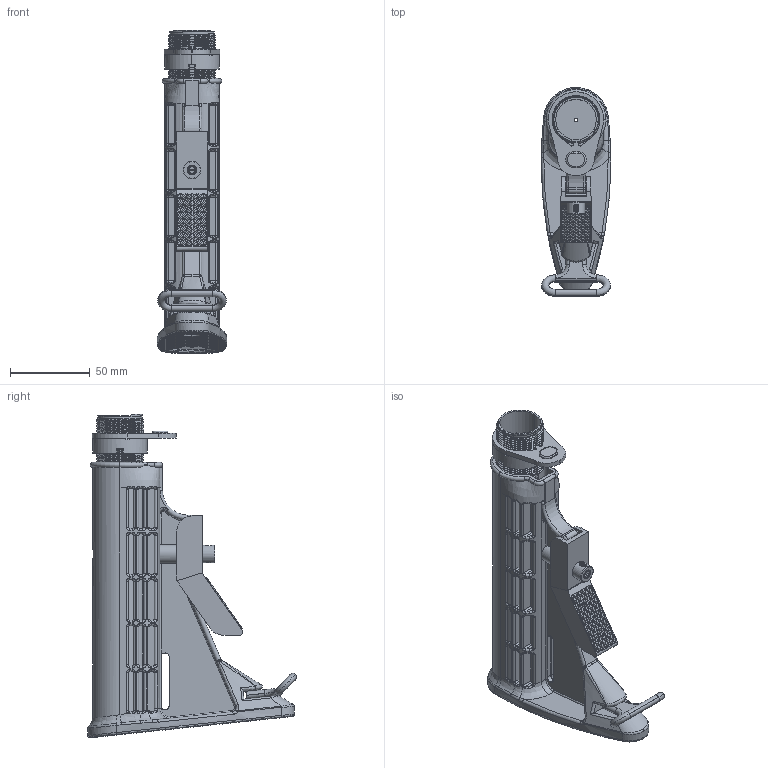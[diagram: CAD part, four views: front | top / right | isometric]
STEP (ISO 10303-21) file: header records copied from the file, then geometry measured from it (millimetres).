
FILE_DESCRIPTION (( 'STEP AP214' ), '1' );
FILE_NAME ('User Library-Telescopic Stock_1.STEP', '2013-05-22T15:48:38', ( 'Asher' ), ( '' ), 'SwSTEP 2.0', 'SolidWorks 2013', '' );
FILE_SCHEMA (( 'AUTOMOTIVE_DESIGN' ));
Length unit declared in the file: inch
Products named in the file (12): User Library-Telescopic Stock_Telescopic Stock Tube1_1; User Library-Telescopic Stock_Telescopic Stock Swivel Screw1_1; User Library-Telescopic Stock_Stock Bolt1_1; User Library-Telescopic Stock_Telescopic Stock Spring_Installed1_1; User Library-Telescopic Stock_1; User Library-Telescopic Stock_Stock Bolt Nut1_1; User Library-Telescopic Stock_Telescopic Stock Swivel1_1; User Library-Telescopic Stock_5310-917-1154_1; User Library-Telescopic Stock_Telescopic Stock_Default_As Machined_1_1; User Library-Telescopic Stock_Telescopic stock Roll Pin1_1; User Library-Telescopic Stock_Telescopic Stock Lever1_1; User Library-Telescopic Stock_1005-914-2943_1
Assembly tree (11 placements, depth 2):
  User Library-Telescopic Stock_1
    User Library-Telescopic Stock_Telescopic Stock Spring_Installed1_1
    User Library-Telescopic Stock_Stock Bolt1_1
    User Library-Telescopic Stock_Telescopic Stock Swivel Screw1_1
    User Library-Telescopic Stock_Telescopic Stock Tube1_1
    User Library-Telescopic Stock_1005-914-2943_1
    User Library-Telescopic Stock_Telescopic Stock Lever1_1
    User Library-Telescopic Stock_Telescopic stock Roll Pin1_1
    User Library-Telescopic Stock_Telescopic Stock_Default_As Machined_1_1
    User Library-Telescopic Stock_5310-917-1154_1
    User Library-Telescopic Stock_Telescopic Stock Swivel1_1
    User Library-Telescopic Stock_Stock Bolt Nut1_1
Bounding box: 43.56 x 130.88 x 202.7 mm (x, y, z)
Volume: 180797.3 mm3; surface area: 124908.4 mm2
Topology: 11 solids, 11 shells, 4888 faces, 12451 edges, 8160 vertices
Faces by surface type: plane 3748, cylinder 619, bspline 328, torus 148, cone 39, sphere 6
Entity records: 259785 total; most frequent: CARTESIAN_POINT 147494, ORIENTED_EDGE 24898, DIRECTION 19470, EDGE_CURVE 12449, VECTOR 8876, LINE 8876, VERTEX_POINT 8159, EDGE_LOOP 5492
